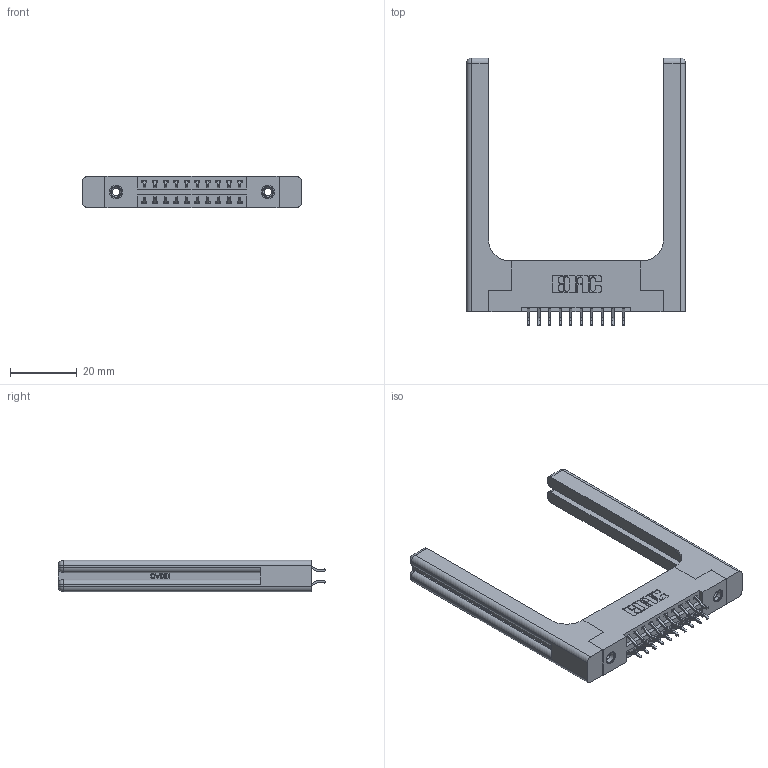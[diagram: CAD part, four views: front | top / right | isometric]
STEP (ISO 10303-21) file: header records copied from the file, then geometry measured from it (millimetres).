
FILE_DESCRIPTION (( 'STEP AP203' ), '1' );
FILE_NAME ('396-020-556-258.STEP', '2019-10-30T03:31:48', ( '' ), ( '' ), 'SwSTEP 2.0', 'SolidWorks 2016', '' );
FILE_SCHEMA (( 'CONFIG_CONTROL_DESIGN' ));
Length unit declared in the file: inch
Products named in the file (5): 346-220-058_345-220-058; 345-250-001_345-250-001-102; 345-292-001_556 Tail; 346 Part_Flush Mounting Lugs - 0.156 Dia-TH; 396-020-556-258
Assembly tree (25 placements, depth 2):
  396-020-556-258
    346 Part_Flush Mounting Lugs - 0.156 Dia-TH
    345-292-001_556 Tail  x20
    345-250-001_345-250-001-102  x2
    346-220-058_345-220-058  x2
Bounding box: 65.81 x 80.53 x 9.4 mm (x, y, z)
Volume: 13662.3 mm3; surface area: 12929.7 mm2
Topology: 25 solids, 25 shells, 1538 faces, 4455 edges, 2922 vertices
Faces by surface type: plane 1004, cylinder 474, bspline 36, cone 12, sphere 8, torus 4
Entity records: 16236 total; most frequent: CARTESIAN_POINT 3741, ORIENTED_EDGE 2460, DIRECTION 2270, EDGE_CURVE 1230, LINE 958, VECTOR 958, VERTEX_POINT 810, AXIS2_PLACEMENT_3D 656
